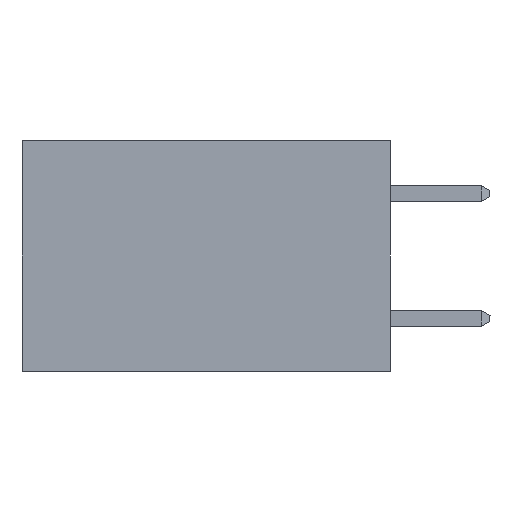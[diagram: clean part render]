
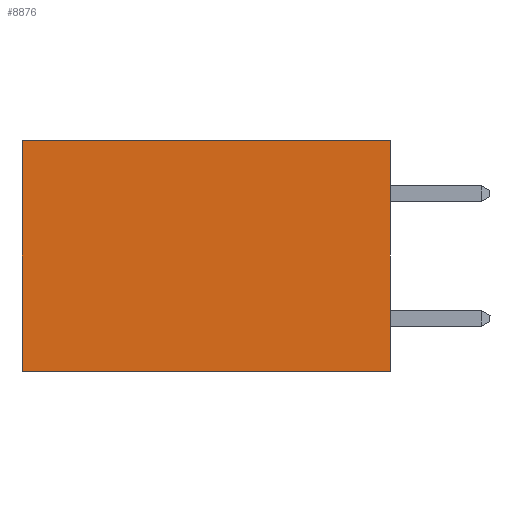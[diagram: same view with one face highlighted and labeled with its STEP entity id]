
A CAD part, left-side view. The second image highlights one B-rep face of the part: STEP entity #8876.
In plain terms, the highlighted planar face has unit normal (-1, 0, 0).
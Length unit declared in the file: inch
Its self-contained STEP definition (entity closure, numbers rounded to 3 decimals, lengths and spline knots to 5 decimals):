
#199 = EDGE_CURVE ( 'NONE', #1955, #5838, #6065, .T. ) ;
#403 = ORIENTED_EDGE ( 'NONE', *, *, #199, .T. ) ;
#491 = PLANE ( 'NONE',  #8830 ) ;
#529 = DIRECTION ( 'NONE',  ( 0., 0., -1. ) ) ;
#570 = ORIENTED_EDGE ( 'NONE', *, *, #3466, .F. ) ;
#1261 = ORIENTED_EDGE ( 'NONE', *, *, #3423, .F. ) ;
#1790 = VECTOR ( 'NONE', #4648, 39.37008 ) ;
#1911 = LINE ( 'NONE', #5090, #9181 ) ;
#1955 = VERTEX_POINT ( 'NONE', #3595 ) ;
#2180 = ORIENTED_EDGE ( 'NONE', *, *, #5616, .T. ) ;
#2406 = CARTESIAN_POINT ( 'NONE',  ( 0.277, 0., -0.37 ) ) ;
#2987 = LINE ( 'NONE', #7761, #4765 ) ;
#3273 = LINE ( 'NONE', #6143, #3517 ) ;
#3423 = EDGE_CURVE ( 'NONE', #5345, #5838, #1911, .T. ) ;
#3466 = EDGE_CURVE ( 'NONE', #7198, #5345, #3273, .T. ) ;
#3517 = VECTOR ( 'NONE', #6237, 39.37008 ) ;
#3595 = CARTESIAN_POINT ( 'NONE',  ( 0.277, 0.59, 0. ) ) ;
#3908 = FACE_OUTER_BOUND ( 'NONE', #5885, .T. ) ;
#4234 = DIRECTION ( 'NONE',  ( 0., 1., 0. ) ) ;
#4648 = DIRECTION ( 'NONE',  ( 0., 0., -1. ) ) ;
#4765 = VECTOR ( 'NONE', #4915, 39.37008 ) ;
#4915 = DIRECTION ( 'NONE',  ( 0., 1., 0. ) ) ;
#5090 = CARTESIAN_POINT ( 'NONE',  ( 0.277, 0., -0.37 ) ) ;
#5166 = DIRECTION ( 'NONE',  ( 1., 0., 0. ) ) ;
#5345 = VERTEX_POINT ( 'NONE', #2406 ) ;
#5616 = EDGE_CURVE ( 'NONE', #7198, #1955, #2987, .T. ) ;
#5838 = VERTEX_POINT ( 'NONE', #8681 ) ;
#5885 = EDGE_LOOP ( 'NONE', ( #403, #1261, #570, #2180 ) ) ;
#6065 = LINE ( 'NONE', #9075, #1790 ) ;
#6143 = CARTESIAN_POINT ( 'NONE',  ( 0.277, 0., -0.37 ) ) ;
#6237 = DIRECTION ( 'NONE',  ( 0., 0., -1. ) ) ;
#6678 = CARTESIAN_POINT ( 'NONE',  ( 0.277, 0., 0. ) ) ;
#7198 = VERTEX_POINT ( 'NONE', #6678 ) ;
#7761 = CARTESIAN_POINT ( 'NONE',  ( 0.277, 0., 0. ) ) ;
#8660 = CARTESIAN_POINT ( 'NONE',  ( 0.277, 0., -0.37 ) ) ;
#8681 = CARTESIAN_POINT ( 'NONE',  ( 0.277, 0.59, -0.37 ) ) ;
#8830 = AXIS2_PLACEMENT_3D ( 'NONE', #8660, #5166, #529 ) ;
#8876 = ADVANCED_FACE ( 'NONE', ( #3908 ), #491, .F. ) ;
#9075 = CARTESIAN_POINT ( 'NONE',  ( 0.277, 0.59, -0.37 ) ) ;
#9181 = VECTOR ( 'NONE', #4234, 39.37008 ) ;
